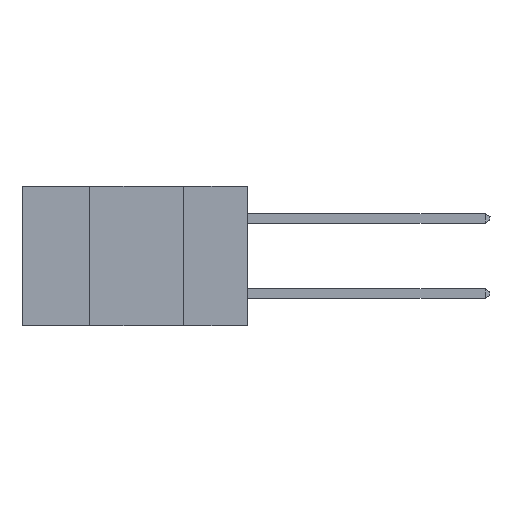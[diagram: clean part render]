
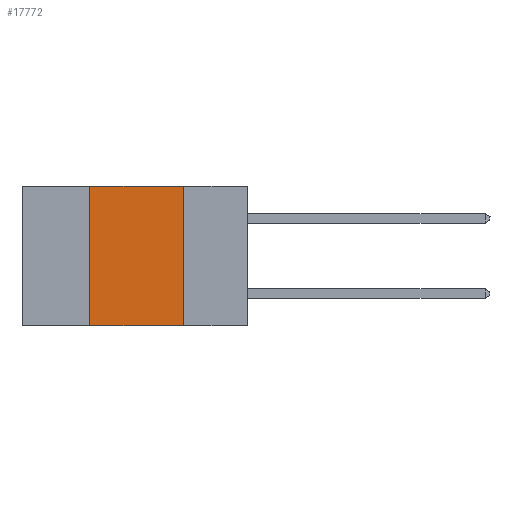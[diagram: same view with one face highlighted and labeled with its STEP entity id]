
A CAD part, left-side view. The second image highlights one B-rep face of the part: STEP entity #17772.
In plain terms, the highlighted planar face has unit normal (-1, 0, 0).
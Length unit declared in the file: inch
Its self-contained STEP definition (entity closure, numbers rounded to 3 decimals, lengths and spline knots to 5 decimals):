
#625 = CARTESIAN_POINT ( 'NONE',  ( 0., 0.6, 0. ) ) ;
#2128 = VECTOR ( 'NONE', #18675, 39.37008 ) ;
#2245 = PLANE ( 'NONE',  #4337 ) ;
#2838 = CARTESIAN_POINT ( 'NONE',  ( 0., 0.42, 0. ) ) ;
#2882 = VECTOR ( 'NONE', #14171, 39.37008 ) ;
#2986 = EDGE_CURVE ( 'NONE', #7967, #8171, #12600, .T. ) ;
#3782 = DIRECTION ( 'NONE',  ( 1., 0., 0. ) ) ;
#4244 = CARTESIAN_POINT ( 'NONE',  ( 0., 0.17, 0. ) ) ;
#4262 = ORIENTED_EDGE ( 'NONE', *, *, #2986, .F. ) ;
#4337 = AXIS2_PLACEMENT_3D ( 'NONE', #625, #3782, #8047 ) ;
#5966 = LINE ( 'NONE', #10429, #11906 ) ;
#7316 = EDGE_CURVE ( 'NONE', #13546, #7967, #8482, .T. ) ;
#7967 = VERTEX_POINT ( 'NONE', #2838 ) ;
#8047 = DIRECTION ( 'NONE',  ( 0., 0., -1. ) ) ;
#8171 = VERTEX_POINT ( 'NONE', #4244 ) ;
#8482 = LINE ( 'NONE', #18731, #2882 ) ;
#8584 = CARTESIAN_POINT ( 'NONE',  ( 0., 0.42, -0.37 ) ) ;
#8864 = VERTEX_POINT ( 'NONE', #12317 ) ;
#9816 = ORIENTED_EDGE ( 'NONE', *, *, #10201, .F. ) ;
#9967 = CARTESIAN_POINT ( 'NONE',  ( 0., 0.6, -0.37 ) ) ;
#10201 = EDGE_CURVE ( 'NONE', #8171, #8864, #5966, .T. ) ;
#10429 = CARTESIAN_POINT ( 'NONE',  ( 0., 0.17, -0.37 ) ) ;
#11349 = DIRECTION ( 'NONE',  ( 0., -1., 0. ) ) ;
#11906 = VECTOR ( 'NONE', #17900, 39.37008 ) ;
#12317 = CARTESIAN_POINT ( 'NONE',  ( 0., 0.17, -0.37 ) ) ;
#12574 = FACE_OUTER_BOUND ( 'NONE', #16763, .T. ) ;
#12600 = LINE ( 'NONE', #17111, #15287 ) ;
#12849 = LINE ( 'NONE', #9967, #2128 ) ;
#13139 = ORIENTED_EDGE ( 'NONE', *, *, #7316, .F. ) ;
#13546 = VERTEX_POINT ( 'NONE', #8584 ) ;
#14171 = DIRECTION ( 'NONE',  ( 0., 0., 1. ) ) ;
#14565 = EDGE_CURVE ( 'NONE', #13546, #8864, #12849, .T. ) ;
#15287 = VECTOR ( 'NONE', #11349, 39.37008 ) ;
#16763 = EDGE_LOOP ( 'NONE', ( #9816, #4262, #13139, #18813 ) ) ;
#17111 = CARTESIAN_POINT ( 'NONE',  ( 0., 0.6, 0. ) ) ;
#17772 = ADVANCED_FACE ( 'NONE', ( #12574 ), #2245, .F. ) ;
#17900 = DIRECTION ( 'NONE',  ( 0., 0., -1. ) ) ;
#18675 = DIRECTION ( 'NONE',  ( 0., -1., 0. ) ) ;
#18731 = CARTESIAN_POINT ( 'NONE',  ( 0., 0.42, -0.37 ) ) ;
#18813 = ORIENTED_EDGE ( 'NONE', *, *, #14565, .T. ) ;
